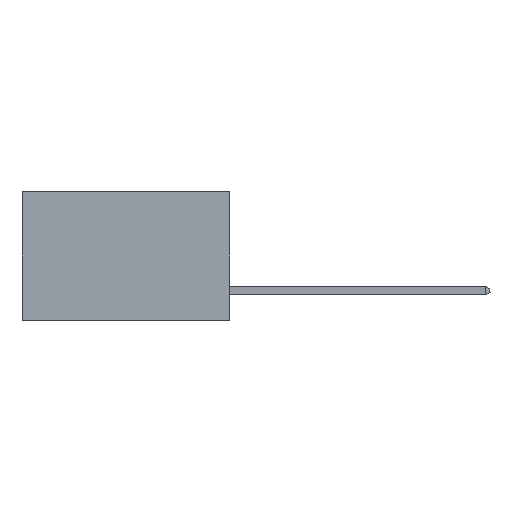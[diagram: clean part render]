
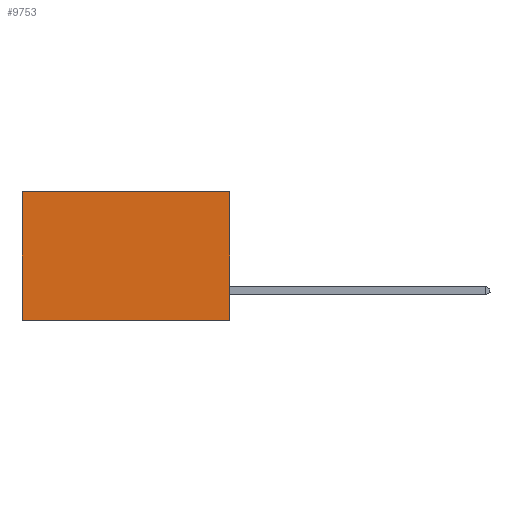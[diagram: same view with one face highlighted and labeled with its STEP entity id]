
A CAD part, left-side view. The second image highlights one B-rep face of the part: STEP entity #9753.
In plain terms, the highlighted planar face has unit normal (-1, 0, 0).
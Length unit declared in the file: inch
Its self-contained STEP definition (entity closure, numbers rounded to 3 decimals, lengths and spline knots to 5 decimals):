
#171 = DIRECTION ( 'NONE',  ( 0., 1., 0. ) ) ;
#435 = PLANE ( 'NONE',  #16202 ) ;
#651 = VECTOR ( 'NONE', #8088, 39.37008 ) ;
#2693 = CARTESIAN_POINT ( 'NONE',  ( 0.298, 0.6, -0.37 ) ) ;
#3437 = EDGE_LOOP ( 'NONE', ( #12681, #3583, #19911, #4322 ) ) ;
#3583 = ORIENTED_EDGE ( 'NONE', *, *, #24359, .F. ) ;
#4307 = DIRECTION ( 'NONE',  ( 0., 1., 0. ) ) ;
#4322 = ORIENTED_EDGE ( 'NONE', *, *, #11755, .T. ) ;
#5609 = VECTOR ( 'NONE', #4307, 39.37008 ) ;
#5861 = LINE ( 'NONE', #8016, #651 ) ;
#6164 = DIRECTION ( 'NONE',  ( 0., 0., -1. ) ) ;
#7443 = VECTOR ( 'NONE', #171, 39.37008 ) ;
#7962 = CARTESIAN_POINT ( 'NONE',  ( 0.298, 0., 0. ) ) ;
#8016 = CARTESIAN_POINT ( 'NONE',  ( 0.298, 0., 0. ) ) ;
#8088 = DIRECTION ( 'NONE',  ( 0., 0., -1. ) ) ;
#8354 = VECTOR ( 'NONE', #6164, 39.37008 ) ;
#9062 = FACE_OUTER_BOUND ( 'NONE', #3437, .T. ) ;
#9753 = ADVANCED_FACE ( 'NONE', ( #9062 ), #435, .F. ) ;
#11755 = EDGE_CURVE ( 'NONE', #23894, #19138, #19784, .T. ) ;
#11921 = CARTESIAN_POINT ( 'NONE',  ( 0.298, 0., 0. ) ) ;
#12681 = ORIENTED_EDGE ( 'NONE', *, *, #16751, .T. ) ;
#14170 = DIRECTION ( 'NONE',  ( 0., 0., -1. ) ) ;
#14831 = LINE ( 'NONE', #21651, #8354 ) ;
#16202 = AXIS2_PLACEMENT_3D ( 'NONE', #24138, #18102, #14170 ) ;
#16751 = EDGE_CURVE ( 'NONE', #19138, #19205, #14831, .T. ) ;
#18102 = DIRECTION ( 'NONE',  ( 1., 0., 0. ) ) ;
#18343 = CARTESIAN_POINT ( 'NONE',  ( 0.298, 0.6, 0. ) ) ;
#19138 = VERTEX_POINT ( 'NONE', #18343 ) ;
#19205 = VERTEX_POINT ( 'NONE', #2693 ) ;
#19784 = LINE ( 'NONE', #7962, #7443 ) ;
#19911 = ORIENTED_EDGE ( 'NONE', *, *, #25268, .F. ) ;
#20483 = CARTESIAN_POINT ( 'NONE',  ( 0.298, 0., -0.37 ) ) ;
#21315 = LINE ( 'NONE', #21931, #5609 ) ;
#21651 = CARTESIAN_POINT ( 'NONE',  ( 0.298, 0.6, 0. ) ) ;
#21931 = CARTESIAN_POINT ( 'NONE',  ( 0.298, 0., -0.37 ) ) ;
#23452 = VERTEX_POINT ( 'NONE', #20483 ) ;
#23894 = VERTEX_POINT ( 'NONE', #11921 ) ;
#24138 = CARTESIAN_POINT ( 'NONE',  ( 0.298, 0., 0. ) ) ;
#24359 = EDGE_CURVE ( 'NONE', #23452, #19205, #21315, .T. ) ;
#25268 = EDGE_CURVE ( 'NONE', #23894, #23452, #5861, .T. ) ;
